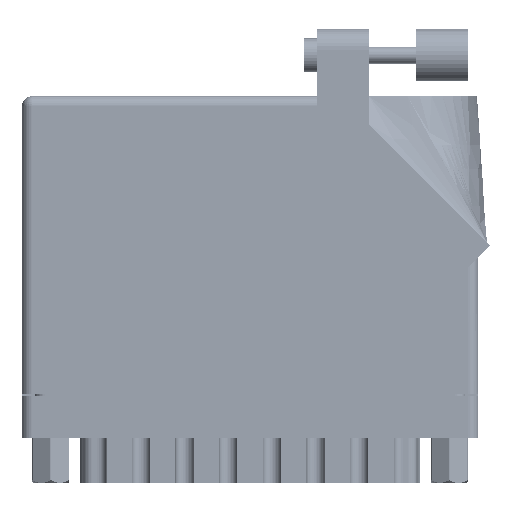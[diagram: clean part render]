
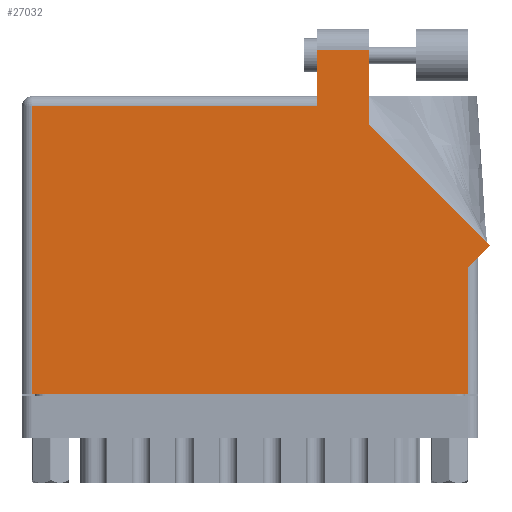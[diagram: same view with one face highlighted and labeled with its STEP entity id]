
A CAD part, front view. The second image highlights one B-rep face of the part: STEP entity #27032.
In plain terms, the highlighted face is planar.
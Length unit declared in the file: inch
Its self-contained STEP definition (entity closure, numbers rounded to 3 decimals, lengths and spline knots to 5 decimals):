
#6980 = EDGE_CURVE ( 'NONE', #42137, #68346, #72558, .T. ) ;
#7730 = LINE ( 'NONE', #54671, #71132 ) ;
#9578 = VECTOR ( 'NONE', #52401, 39.37008 ) ;
#11380 = ORIENTED_EDGE ( 'NONE', *, *, #18064, .T. ) ;
#11562 = LINE ( 'NONE', #17390, #51105 ) ;
#15092 = LINE ( 'NONE', #35899, #83670 ) ;
#15898 = AXIS2_PLACEMENT_3D ( 'NONE', #45538, #79180, #64969 ) ;
#16093 = DIRECTION ( 'NONE',  ( 0.707, 0.707, 0. ) ) ;
#17390 = CARTESIAN_POINT ( 'NONE',  ( 2.78871, 0.88571, 0. ) ) ;
#18064 = EDGE_CURVE ( 'NONE', #79800, #35706, #59245, .T. ) ;
#18702 = ORIENTED_EDGE ( 'NONE', *, *, #41631, .T. ) ;
#18756 = PLANE ( 'NONE',  #15898 ) ;
#27032 = ADVANCED_FACE ( 'NONE', ( #32204 ), #18756, .F. ) ;
#27105 = EDGE_CURVE ( 'NONE', #55214, #58441, #71628, .T. ) ;
#27928 = CARTESIAN_POINT ( 'NONE',  ( 0.062, 1.713, 0. ) ) ;
#29088 = ORIENTED_EDGE ( 'NONE', *, *, #27105, .T. ) ;
#29409 = LINE ( 'NONE', #65167, #9578 ) ;
#29933 = DIRECTION ( 'NONE',  ( -0.707, 0.707, 0. ) ) ;
#32204 = FACE_OUTER_BOUND ( 'NONE', #46771, .T. ) ;
#35706 = VERTEX_POINT ( 'NONE', #66590 ) ;
#35899 = CARTESIAN_POINT ( 'NONE',  ( 2.718, 0.815, 0. ) ) ;
#36447 = CARTESIAN_POINT ( 'NONE',  ( 2.656, 0.753, 0. ) ) ;
#38941 = ORIENTED_EDGE ( 'NONE', *, *, #70973, .T. ) ;
#39022 = DIRECTION ( 'NONE',  ( 1., 0., 0. ) ) ;
#41631 = EDGE_CURVE ( 'NONE', #51965, #54899, #15092, .T. ) ;
#42137 = VERTEX_POINT ( 'NONE', #86001 ) ;
#42187 = VERTEX_POINT ( 'NONE', #27928 ) ;
#42236 = EDGE_CURVE ( 'NONE', #58441, #42187, #7730, .T. ) ;
#42285 = ORIENTED_EDGE ( 'NONE', *, *, #42236, .T. ) ;
#43398 = CARTESIAN_POINT ( 'NONE',  ( 1.758, 2.05, 0. ) ) ;
#45538 = CARTESIAN_POINT ( 'NONE',  ( 0., 1.775, 0. ) ) ;
#46055 = VECTOR ( 'NONE', #73888, 39.37008 ) ;
#46771 = EDGE_LOOP ( 'NONE', ( #11380, #85355, #29088, #42285, #38941, #57160, #47657, #18702, #73549 ) ) ;
#47657 = ORIENTED_EDGE ( 'NONE', *, *, #67720, .T. ) ;
#47739 = EDGE_CURVE ( 'NONE', #35706, #55214, #73408, .T. ) ;
#51105 = VECTOR ( 'NONE', #29933, 39.37008 ) ;
#51965 = VERTEX_POINT ( 'NONE', #36447 ) ;
#52401 = DIRECTION ( 'NONE',  ( 0., 1., 0. ) ) ;
#52982 = VECTOR ( 'NONE', #79455, 39.37008 ) ;
#53988 = EDGE_CURVE ( 'NONE', #54899, #79800, #11562, .T. ) ;
#54671 = CARTESIAN_POINT ( 'NONE',  ( 0., 1.713, 0. ) ) ;
#54899 = VERTEX_POINT ( 'NONE', #66943 ) ;
#55214 = VERTEX_POINT ( 'NONE', #43398 ) ;
#55525 = DIRECTION ( 'NONE',  ( -1., 0., 0. ) ) ;
#57160 = ORIENTED_EDGE ( 'NONE', *, *, #6980, .T. ) ;
#58441 = VERTEX_POINT ( 'NONE', #75636 ) ;
#59245 = LINE ( 'NONE', #82359, #64418 ) ;
#59414 = CARTESIAN_POINT ( 'NONE',  ( 1.758, 2.05, 0. ) ) ;
#59930 = VECTOR ( 'NONE', #66099, 39.37008 ) ;
#60261 = CARTESIAN_POINT ( 'NONE',  ( 1.758, 1.775, 0. ) ) ;
#61723 = CARTESIAN_POINT ( 'NONE',  ( 0.062, 0., 0. ) ) ;
#64418 = VECTOR ( 'NONE', #76252, 39.37008 ) ;
#64969 = DIRECTION ( 'NONE',  ( -1., 0., 0. ) ) ;
#65167 = CARTESIAN_POINT ( 'NONE',  ( 2.656, 0.815, 0. ) ) ;
#65275 = CARTESIAN_POINT ( 'NONE',  ( 2.656, 0., 0. ) ) ;
#65705 = CARTESIAN_POINT ( 'NONE',  ( 0., 0., 0. ) ) ;
#66099 = DIRECTION ( 'NONE',  ( -1., 0., 0. ) ) ;
#66590 = CARTESIAN_POINT ( 'NONE',  ( 2.065, 2.05, 0. ) ) ;
#66943 = CARTESIAN_POINT ( 'NONE',  ( 2.78871, 0.88571, 0. ) ) ;
#67720 = EDGE_CURVE ( 'NONE', #68346, #51965, #29409, .T. ) ;
#68346 = VERTEX_POINT ( 'NONE', #65275 ) ;
#70973 = EDGE_CURVE ( 'NONE', #42187, #42137, #81334, .T. ) ;
#71132 = VECTOR ( 'NONE', #55525, 39.37008 ) ;
#71628 = LINE ( 'NONE', #60261, #52982 ) ;
#72558 = LINE ( 'NONE', #65705, #78819 ) ;
#73408 = LINE ( 'NONE', #59414, #59930 ) ;
#73549 = ORIENTED_EDGE ( 'NONE', *, *, #53988, .T. ) ;
#73888 = DIRECTION ( 'NONE',  ( 0., -1., 0. ) ) ;
#75636 = CARTESIAN_POINT ( 'NONE',  ( 1.758, 1.713, 0. ) ) ;
#76252 = DIRECTION ( 'NONE',  ( 0., 1., 0. ) ) ;
#78819 = VECTOR ( 'NONE', #39022, 39.37008 ) ;
#79180 = DIRECTION ( 'NONE',  ( 0., 0., -1. ) ) ;
#79455 = DIRECTION ( 'NONE',  ( 0., -1., 0. ) ) ;
#79800 = VERTEX_POINT ( 'NONE', #86110 ) ;
#81334 = LINE ( 'NONE', #61723, #46055 ) ;
#82359 = CARTESIAN_POINT ( 'NONE',  ( 2.065, 1.60942, 0. ) ) ;
#83670 = VECTOR ( 'NONE', #16093, 39.37008 ) ;
#85355 = ORIENTED_EDGE ( 'NONE', *, *, #47739, .T. ) ;
#86001 = CARTESIAN_POINT ( 'NONE',  ( 0.062, 0., 0. ) ) ;
#86110 = CARTESIAN_POINT ( 'NONE',  ( 2.065, 1.60942, 0. ) ) ;
